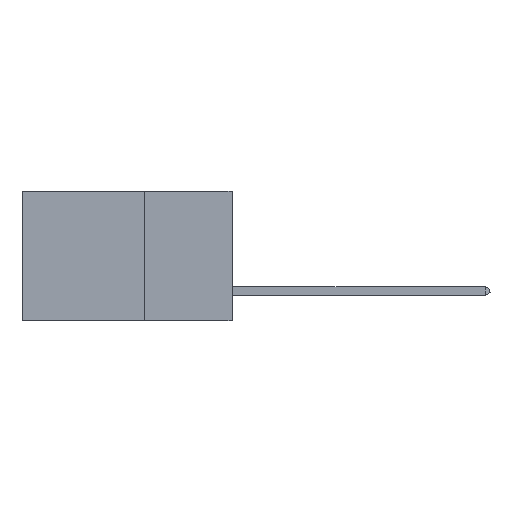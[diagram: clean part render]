
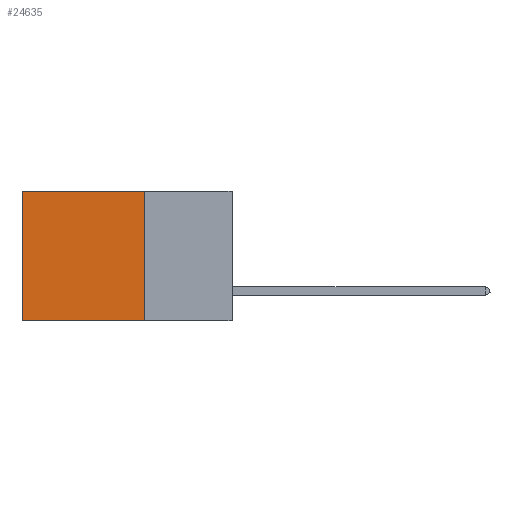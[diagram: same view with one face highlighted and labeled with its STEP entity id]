
A CAD part, left-side view. The second image highlights one B-rep face of the part: STEP entity #24635.
In plain terms, the highlighted planar face has unit normal (-1, 0, 0).
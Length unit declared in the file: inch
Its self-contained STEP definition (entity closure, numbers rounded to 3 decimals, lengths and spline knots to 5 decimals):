
#1377 = CARTESIAN_POINT ( 'NONE',  ( 0.2875, 0.6, 0. ) ) ;
#6803 = DIRECTION ( 'NONE',  ( 1., 0., 0. ) ) ;
#7179 = VECTOR ( 'NONE', #21715, 39.37008 ) ;
#8577 = ORIENTED_EDGE ( 'NONE', *, *, #32074, .T. ) ;
#8632 = LINE ( 'NONE', #26713, #14029 ) ;
#9537 = EDGE_CURVE ( 'NONE', #25109, #23413, #8632, .T. ) ;
#9663 = VERTEX_POINT ( 'NONE', #34981 ) ;
#12275 = ORIENTED_EDGE ( 'NONE', *, *, #38034, .T. ) ;
#13311 = PLANE ( 'NONE',  #40262 ) ;
#13580 = ORIENTED_EDGE ( 'NONE', *, *, #29653, .F. ) ;
#14029 = VECTOR ( 'NONE', #27837, 39.37008 ) ;
#15599 = LINE ( 'NONE', #29076, #22027 ) ;
#16530 = DIRECTION ( 'NONE',  ( 0., 1., 0. ) ) ;
#17194 = CARTESIAN_POINT ( 'NONE',  ( 0.2875, 0.25, 0. ) ) ;
#18453 = VERTEX_POINT ( 'NONE', #1377 ) ;
#20392 = CARTESIAN_POINT ( 'NONE',  ( 0.2875, 0.25, -0.37 ) ) ;
#21715 = DIRECTION ( 'NONE',  ( 0., 0., -1. ) ) ;
#22027 = VECTOR ( 'NONE', #16530, 39.37008 ) ;
#22550 = FACE_OUTER_BOUND ( 'NONE', #22613, .T. ) ;
#22613 = EDGE_LOOP ( 'NONE', ( #8577, #13580, #29985, #12275 ) ) ;
#23413 = VERTEX_POINT ( 'NONE', #20392 ) ;
#23956 = LINE ( 'NONE', #27896, #7179 ) ;
#24635 = ADVANCED_FACE ( 'NONE', ( #22550 ), #13311, .F. ) ;
#25109 = VERTEX_POINT ( 'NONE', #17194 ) ;
#26047 = DIRECTION ( 'NONE',  ( 0., 0., -1. ) ) ;
#26713 = CARTESIAN_POINT ( 'NONE',  ( 0.2875, 0.25, 0. ) ) ;
#27837 = DIRECTION ( 'NONE',  ( 0., 0., -1. ) ) ;
#27896 = CARTESIAN_POINT ( 'NONE',  ( 0.2875, 0.6, 0. ) ) ;
#28565 = CARTESIAN_POINT ( 'NONE',  ( 0.2875, 0.25, 0. ) ) ;
#29076 = CARTESIAN_POINT ( 'NONE',  ( 0.2875, 0.25, 0. ) ) ;
#29653 = EDGE_CURVE ( 'NONE', #23413, #9663, #38281, .T. ) ;
#29985 = ORIENTED_EDGE ( 'NONE', *, *, #9537, .F. ) ;
#32074 = EDGE_CURVE ( 'NONE', #18453, #9663, #23956, .T. ) ;
#32325 = DIRECTION ( 'NONE',  ( 0., 1., 0. ) ) ;
#34981 = CARTESIAN_POINT ( 'NONE',  ( 0.2875, 0.6, -0.37 ) ) ;
#38034 = EDGE_CURVE ( 'NONE', #25109, #18453, #15599, .T. ) ;
#38209 = CARTESIAN_POINT ( 'NONE',  ( 0.2875, 0.25, -0.37 ) ) ;
#38281 = LINE ( 'NONE', #38209, #39267 ) ;
#39267 = VECTOR ( 'NONE', #32325, 39.37008 ) ;
#40262 = AXIS2_PLACEMENT_3D ( 'NONE', #28565, #6803, #26047 ) ;
